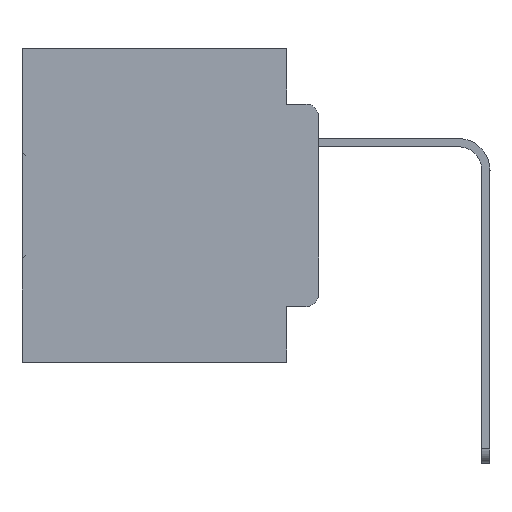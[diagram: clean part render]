
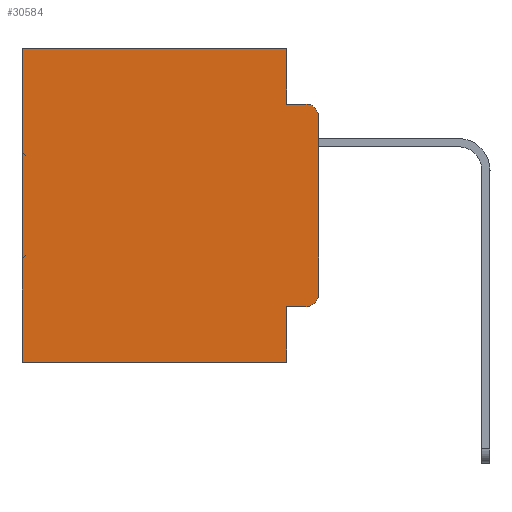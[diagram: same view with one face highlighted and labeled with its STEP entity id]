
A CAD part, left-side view. The second image highlights one B-rep face of the part: STEP entity #30584.
In plain terms, the highlighted planar face has unit normal (-1, 0, 0).
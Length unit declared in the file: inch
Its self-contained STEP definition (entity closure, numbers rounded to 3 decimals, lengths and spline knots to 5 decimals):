
#606 = DIRECTION ( 'NONE',  ( 0., -1., 0. ) ) ;
#1373 = CARTESIAN_POINT ( 'NONE',  ( 0.298, 0.051, -0.4115 ) ) ;
#2023 = DIRECTION ( 'NONE',  ( 0., 1., 0. ) ) ;
#3209 = AXIS2_PLACEMENT_3D ( 'NONE', #11815, #15572, #10323 ) ;
#4492 = CARTESIAN_POINT ( 'NONE',  ( 0.298, 0., 0. ) ) ;
#4921 = CARTESIAN_POINT ( 'NONE',  ( 0.298, 0.02, -0.4115 ) ) ;
#5372 = LINE ( 'NONE', #4492, #28521 ) ;
#5510 = EDGE_CURVE ( 'NONE', #18986, #27739, #7119, .T. ) ;
#6091 = EDGE_CURVE ( 'NONE', #13703, #11723, #21718, .T. ) ;
#6363 = VECTOR ( 'NONE', #606, 39.37008 ) ;
#6769 = ORIENTED_EDGE ( 'NONE', *, *, #9601, .T. ) ;
#6825 = LINE ( 'NONE', #10893, #33570 ) ;
#6914 = CARTESIAN_POINT ( 'NONE',  ( 0.298, 0., -0.5 ) ) ;
#6935 = VERTEX_POINT ( 'NONE', #18363 ) ;
#7021 = ORIENTED_EDGE ( 'NONE', *, *, #12256, .F. ) ;
#7119 = CIRCLE ( 'NONE', #25287, 0.02 ) ;
#7182 = DIRECTION ( 'NONE',  ( -1., 0., 0. ) ) ;
#7314 = VERTEX_POINT ( 'NONE', #17862 ) ;
#7366 = DIRECTION ( 'NONE',  ( 1., 0., 0. ) ) ;
#7837 = ORIENTED_EDGE ( 'NONE', *, *, #9246, .F. ) ;
#7875 = CARTESIAN_POINT ( 'NONE',  ( 0.298, 0.051, -0.4115 ) ) ;
#7915 = EDGE_LOOP ( 'NONE', ( #7837, #15280, #16291, #10105, #21567, #6769, #14840, #7021, #27789, #18339 ) ) ;
#8151 = VERTEX_POINT ( 'NONE', #10537 ) ;
#8306 = DIRECTION ( 'NONE',  ( 0., 0., -1. ) ) ;
#9175 = CARTESIAN_POINT ( 'NONE',  ( 0.298, 0.051, 0. ) ) ;
#9246 = EDGE_CURVE ( 'NONE', #6935, #27739, #24302, .T. ) ;
#9564 = CARTESIAN_POINT ( 'NONE',  ( 0.298, 0.051, 0. ) ) ;
#9601 = EDGE_CURVE ( 'NONE', #7314, #11723, #32737, .T. ) ;
#9642 = VECTOR ( 'NONE', #8306, 39.37008 ) ;
#10105 = ORIENTED_EDGE ( 'NONE', *, *, #20345, .F. ) ;
#10181 = AXIS2_PLACEMENT_3D ( 'NONE', #12353, #7366, #14877 ) ;
#10323 = DIRECTION ( 'NONE',  ( 0., 0., -1. ) ) ;
#10537 = CARTESIAN_POINT ( 'NONE',  ( 0.298, 0.051, -0.0885 ) ) ;
#10728 = EDGE_CURVE ( 'NONE', #6935, #20781, #18996, .T. ) ;
#10893 = CARTESIAN_POINT ( 'NONE',  ( 0.298, 0.051, 0. ) ) ;
#11723 = VERTEX_POINT ( 'NONE', #25018 ) ;
#11815 = CARTESIAN_POINT ( 'NONE',  ( 0.298, 0.02, -0.1085 ) ) ;
#11934 = VECTOR ( 'NONE', #2023, 39.37008 ) ;
#12256 = EDGE_CURVE ( 'NONE', #24046, #13703, #12703, .T. ) ;
#12353 = CARTESIAN_POINT ( 'NONE',  ( 0.298, 0., 0. ) ) ;
#12462 = CARTESIAN_POINT ( 'NONE',  ( 0.298, 0.02, -0.0885 ) ) ;
#12463 = PLANE ( 'NONE',  #10181 ) ;
#12703 = LINE ( 'NONE', #9175, #18042 ) ;
#12941 = CARTESIAN_POINT ( 'NONE',  ( 0.298, 0.051, -0.5 ) ) ;
#13060 = EDGE_CURVE ( 'NONE', #31768, #7314, #5372, .T. ) ;
#13288 = DIRECTION ( 'NONE',  ( 0., 0., -1. ) ) ;
#13507 = CARTESIAN_POINT ( 'NONE',  ( 0.298, 0., 0. ) ) ;
#13703 = VERTEX_POINT ( 'NONE', #12941 ) ;
#13822 = CARTESIAN_POINT ( 'NONE',  ( 0.298, 0., -0.3915 ) ) ;
#14840 = ORIENTED_EDGE ( 'NONE', *, *, #6091, .F. ) ;
#14877 = DIRECTION ( 'NONE',  ( 0., 0., -1. ) ) ;
#14892 = LINE ( 'NONE', #29443, #6363 ) ;
#15042 = VECTOR ( 'NONE', #19593, 39.37008 ) ;
#15280 = ORIENTED_EDGE ( 'NONE', *, *, #10728, .T. ) ;
#15310 = CARTESIAN_POINT ( 'NONE',  ( 0.298, 0.473, 0. ) ) ;
#15572 = DIRECTION ( 'NONE',  ( -1., 0., 0. ) ) ;
#16291 = ORIENTED_EDGE ( 'NONE', *, *, #31460, .F. ) ;
#17364 = VECTOR ( 'NONE', #28463, 39.37008 ) ;
#17651 = DIRECTION ( 'NONE',  ( 0., 0., -1. ) ) ;
#17862 = CARTESIAN_POINT ( 'NONE',  ( 0.298, 0.473, 0. ) ) ;
#18042 = VECTOR ( 'NONE', #29932, 39.37008 ) ;
#18339 = ORIENTED_EDGE ( 'NONE', *, *, #5510, .T. ) ;
#18363 = CARTESIAN_POINT ( 'NONE',  ( 0.298, 0., -0.1085 ) ) ;
#18986 = VERTEX_POINT ( 'NONE', #4921 ) ;
#18996 = CIRCLE ( 'NONE', #3209, 0.02 ) ;
#19437 = EDGE_CURVE ( 'NONE', #24046, #18986, #26402, .T. ) ;
#19593 = DIRECTION ( 'NONE',  ( 0., -1., 0. ) ) ;
#20181 = CARTESIAN_POINT ( 'NONE',  ( 0.298, 0.02, -0.3915 ) ) ;
#20312 = DIRECTION ( 'NONE',  ( 0., 1., 0. ) ) ;
#20345 = EDGE_CURVE ( 'NONE', #31768, #8151, #6825, .T. ) ;
#20781 = VERTEX_POINT ( 'NONE', #12462 ) ;
#21567 = ORIENTED_EDGE ( 'NONE', *, *, #13060, .T. ) ;
#21718 = LINE ( 'NONE', #6914, #11934 ) ;
#24046 = VERTEX_POINT ( 'NONE', #7875 ) ;
#24302 = LINE ( 'NONE', #13507, #9642 ) ;
#25018 = CARTESIAN_POINT ( 'NONE',  ( 0.298, 0.473, -0.5 ) ) ;
#25287 = AXIS2_PLACEMENT_3D ( 'NONE', #20181, #7182, #17651 ) ;
#26402 = LINE ( 'NONE', #1373, #15042 ) ;
#27739 = VERTEX_POINT ( 'NONE', #13822 ) ;
#27789 = ORIENTED_EDGE ( 'NONE', *, *, #19437, .T. ) ;
#28463 = DIRECTION ( 'NONE',  ( 0., 0., -1. ) ) ;
#28521 = VECTOR ( 'NONE', #20312, 39.37008 ) ;
#29443 = CARTESIAN_POINT ( 'NONE',  ( 0.298, 0.051, -0.0885 ) ) ;
#29561 = FACE_OUTER_BOUND ( 'NONE', #7915, .T. ) ;
#29932 = DIRECTION ( 'NONE',  ( 0., 0., -1. ) ) ;
#30584 = ADVANCED_FACE ( 'NONE', ( #29561 ), #12463, .F. ) ;
#31460 = EDGE_CURVE ( 'NONE', #8151, #20781, #14892, .T. ) ;
#31768 = VERTEX_POINT ( 'NONE', #9564 ) ;
#32737 = LINE ( 'NONE', #15310, #17364 ) ;
#33570 = VECTOR ( 'NONE', #13288, 39.37008 ) ;
